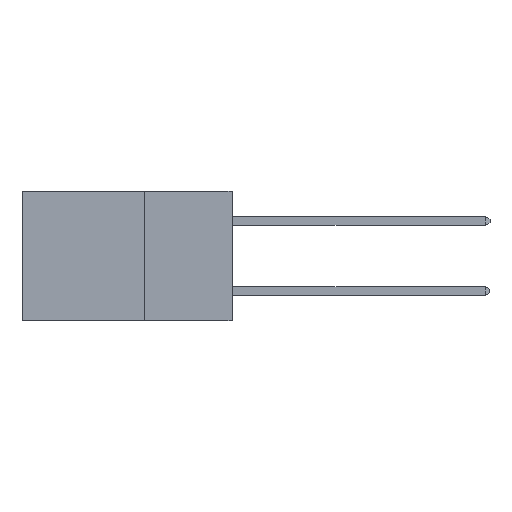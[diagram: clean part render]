
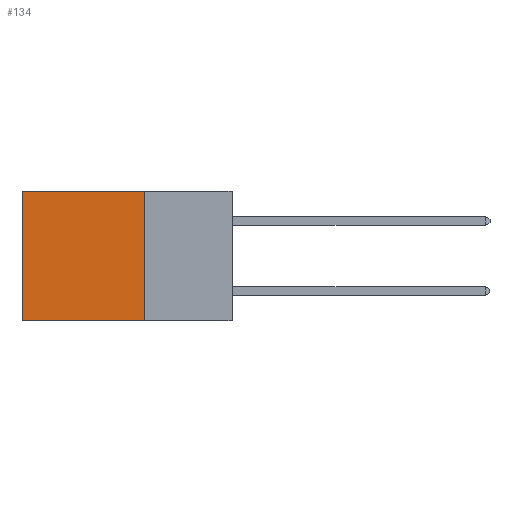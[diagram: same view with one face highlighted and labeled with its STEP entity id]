
A CAD part, left-side view. The second image highlights one B-rep face of the part: STEP entity #134.
In plain terms, the highlighted planar face has unit normal (-1, 0, 0).
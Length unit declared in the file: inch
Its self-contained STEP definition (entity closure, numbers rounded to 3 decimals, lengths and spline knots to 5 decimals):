
#134 = ADVANCED_FACE ( 'NONE', ( #4443 ), #659, .F. ) ;
#567 = CARTESIAN_POINT ( 'NONE',  ( 0.2875, 0.25, 0. ) ) ;
#659 = PLANE ( 'NONE',  #14259 ) ;
#2139 = CARTESIAN_POINT ( 'NONE',  ( 0.2875, 0.25, 0. ) ) ;
#2777 = LINE ( 'NONE', #11353, #15885 ) ;
#2782 = CARTESIAN_POINT ( 'NONE',  ( 0.2875, 0.6, -0.37 ) ) ;
#2910 = VECTOR ( 'NONE', #9559, 39.37008 ) ;
#3667 = DIRECTION ( 'NONE',  ( 0., 0., -1. ) ) ;
#4353 = VECTOR ( 'NONE', #10340, 39.37008 ) ;
#4443 = FACE_OUTER_BOUND ( 'NONE', #5720, .T. ) ;
#4583 = VERTEX_POINT ( 'NONE', #2782 ) ;
#4744 = LINE ( 'NONE', #12634, #4353 ) ;
#5289 = EDGE_CURVE ( 'NONE', #14041, #8114, #4744, .T. ) ;
#5422 = EDGE_CURVE ( 'NONE', #8114, #4583, #2777, .T. ) ;
#5720 = EDGE_LOOP ( 'NONE', ( #12244, #11548, #14359, #15453 ) ) ;
#5913 = VECTOR ( 'NONE', #3667, 39.37008 ) ;
#6292 = DIRECTION ( 'NONE',  ( 1., 0., 0. ) ) ;
#8114 = VERTEX_POINT ( 'NONE', #9322 ) ;
#9322 = CARTESIAN_POINT ( 'NONE',  ( 0.2875, 0.25, -0.37 ) ) ;
#9559 = DIRECTION ( 'NONE',  ( 0., 1., 0. ) ) ;
#10340 = DIRECTION ( 'NONE',  ( 0., 0., -1. ) ) ;
#11251 = CARTESIAN_POINT ( 'NONE',  ( 0.2875, 0.6, 0. ) ) ;
#11353 = CARTESIAN_POINT ( 'NONE',  ( 0.2875, 0.25, -0.37 ) ) ;
#11548 = ORIENTED_EDGE ( 'NONE', *, *, #5422, .F. ) ;
#12056 = CARTESIAN_POINT ( 'NONE',  ( 0.2875, 0.25, 0. ) ) ;
#12101 = EDGE_CURVE ( 'NONE', #14657, #4583, #16477, .T. ) ;
#12244 = ORIENTED_EDGE ( 'NONE', *, *, #12101, .T. ) ;
#12267 = DIRECTION ( 'NONE',  ( 0., 0., -1. ) ) ;
#12634 = CARTESIAN_POINT ( 'NONE',  ( 0.2875, 0.25, 0. ) ) ;
#12662 = DIRECTION ( 'NONE',  ( 0., 1., 0. ) ) ;
#14041 = VERTEX_POINT ( 'NONE', #12056 ) ;
#14259 = AXIS2_PLACEMENT_3D ( 'NONE', #2139, #6292, #12267 ) ;
#14304 = CARTESIAN_POINT ( 'NONE',  ( 0.2875, 0.6, 0. ) ) ;
#14359 = ORIENTED_EDGE ( 'NONE', *, *, #5289, .F. ) ;
#14657 = VERTEX_POINT ( 'NONE', #14304 ) ;
#15453 = ORIENTED_EDGE ( 'NONE', *, *, #15743, .T. ) ;
#15743 = EDGE_CURVE ( 'NONE', #14041, #14657, #15998, .T. ) ;
#15885 = VECTOR ( 'NONE', #12662, 39.37008 ) ;
#15998 = LINE ( 'NONE', #567, #2910 ) ;
#16477 = LINE ( 'NONE', #11251, #5913 ) ;
